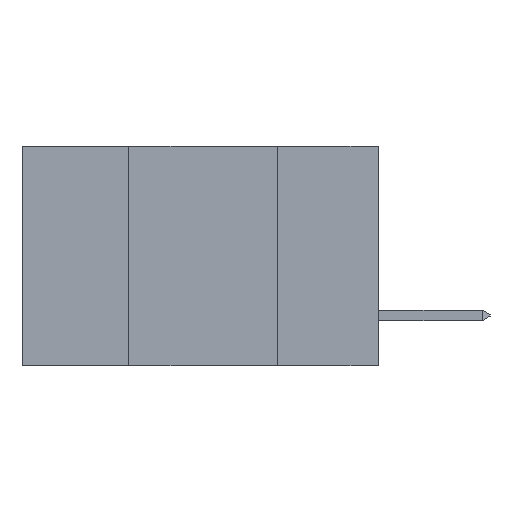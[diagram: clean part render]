
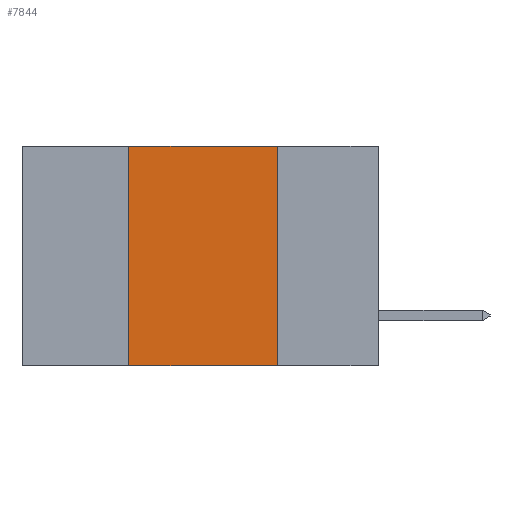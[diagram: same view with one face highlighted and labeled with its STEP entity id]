
A CAD part, left-side view. The second image highlights one B-rep face of the part: STEP entity #7844.
In plain terms, the highlighted planar face has unit normal (-1, 0, 0).
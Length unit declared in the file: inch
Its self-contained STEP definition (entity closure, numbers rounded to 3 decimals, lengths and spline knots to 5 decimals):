
#2093 = LINE ( 'NONE', #3131, #13831 ) ;
#2920 = VERTEX_POINT ( 'NONE', #15393 ) ;
#3131 = CARTESIAN_POINT ( 'NONE',  ( 0., 0.17, -0.37 ) ) ;
#3206 = DIRECTION ( 'NONE',  ( 0., -1., 0. ) ) ;
#5360 = CARTESIAN_POINT ( 'NONE',  ( 0., 0.42, -0.37 ) ) ;
#5635 = VECTOR ( 'NONE', #3206, 39.37008 ) ;
#6017 = CARTESIAN_POINT ( 'NONE',  ( 0., 0.42, -0.37 ) ) ;
#6063 = EDGE_LOOP ( 'NONE', ( #9856, #18957, #6983, #6554 ) ) ;
#6359 = DIRECTION ( 'NONE',  ( 1., 0., 0. ) ) ;
#6554 = ORIENTED_EDGE ( 'NONE', *, *, #11354, .T. ) ;
#6983 = ORIENTED_EDGE ( 'NONE', *, *, #7077, .F. ) ;
#7077 = EDGE_CURVE ( 'NONE', #10458, #14596, #10396, .T. ) ;
#7844 = ADVANCED_FACE ( 'NONE', ( #8111 ), #15992, .F. ) ;
#7849 = VECTOR ( 'NONE', #17278, 39.37008 ) ;
#8111 = FACE_OUTER_BOUND ( 'NONE', #6063, .T. ) ;
#8502 = VERTEX_POINT ( 'NONE', #14432 ) ;
#9856 = ORIENTED_EDGE ( 'NONE', *, *, #11469, .F. ) ;
#10396 = LINE ( 'NONE', #6017, #14153 ) ;
#10458 = VERTEX_POINT ( 'NONE', #5360 ) ;
#10895 = DIRECTION ( 'NONE',  ( 0., 0., 1. ) ) ;
#11093 = DIRECTION ( 'NONE',  ( 0., 0., -1. ) ) ;
#11354 = EDGE_CURVE ( 'NONE', #10458, #8502, #20512, .T. ) ;
#11469 = EDGE_CURVE ( 'NONE', #2920, #8502, #2093, .T. ) ;
#11752 = AXIS2_PLACEMENT_3D ( 'NONE', #12744, #6359, #17605 ) ;
#12744 = CARTESIAN_POINT ( 'NONE',  ( 0., 0.6, 0. ) ) ;
#13831 = VECTOR ( 'NONE', #11093, 39.37008 ) ;
#14153 = VECTOR ( 'NONE', #10895, 39.37008 ) ;
#14421 = CARTESIAN_POINT ( 'NONE',  ( 0., 0.6, 0. ) ) ;
#14432 = CARTESIAN_POINT ( 'NONE',  ( 0., 0.17, -0.37 ) ) ;
#14596 = VERTEX_POINT ( 'NONE', #15682 ) ;
#14722 = LINE ( 'NONE', #14421, #5635 ) ;
#15393 = CARTESIAN_POINT ( 'NONE',  ( 0., 0.17, 0. ) ) ;
#15668 = CARTESIAN_POINT ( 'NONE',  ( 0., 0.6, -0.37 ) ) ;
#15682 = CARTESIAN_POINT ( 'NONE',  ( 0., 0.42, 0. ) ) ;
#15992 = PLANE ( 'NONE',  #11752 ) ;
#17278 = DIRECTION ( 'NONE',  ( 0., -1., 0. ) ) ;
#17605 = DIRECTION ( 'NONE',  ( 0., 0., -1. ) ) ;
#18957 = ORIENTED_EDGE ( 'NONE', *, *, #19244, .F. ) ;
#19244 = EDGE_CURVE ( 'NONE', #14596, #2920, #14722, .T. ) ;
#20512 = LINE ( 'NONE', #15668, #7849 ) ;
